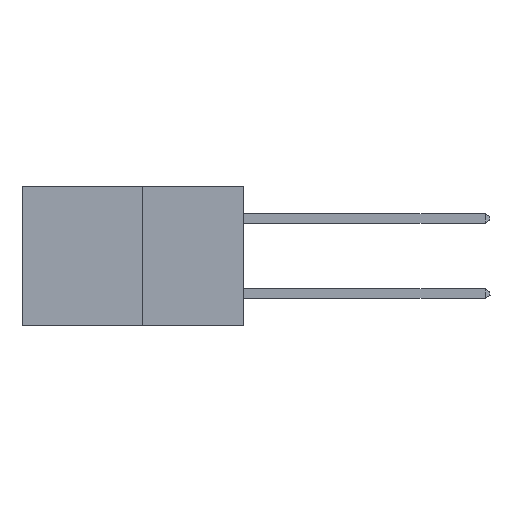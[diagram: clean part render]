
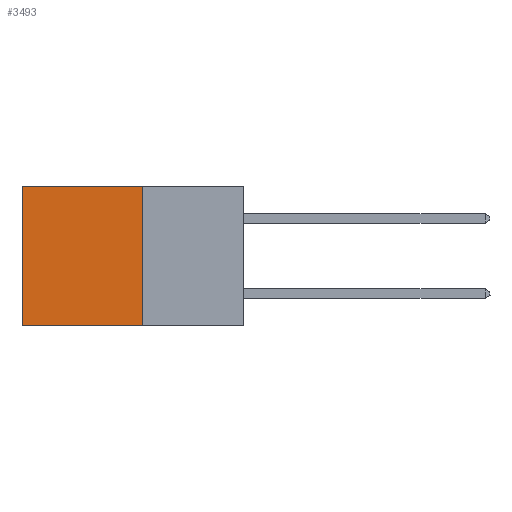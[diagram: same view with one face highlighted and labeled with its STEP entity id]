
A CAD part, left-side view. The second image highlights one B-rep face of the part: STEP entity #3493.
In plain terms, the highlighted planar face has unit normal (-1, 0, 0).
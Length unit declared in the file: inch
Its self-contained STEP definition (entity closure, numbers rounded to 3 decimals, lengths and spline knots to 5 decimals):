
#162 = EDGE_LOOP ( 'NONE', ( #3804, #6174, #7040, #8184 ) ) ;
#469 = CARTESIAN_POINT ( 'NONE',  ( 0.277, 0.27, 0. ) ) ;
#865 = EDGE_CURVE ( 'NONE', #2315, #2094, #4420, .T. ) ;
#960 = CARTESIAN_POINT ( 'NONE',  ( 0.277, 0.27, -0.37 ) ) ;
#1378 = EDGE_CURVE ( 'NONE', #2315, #7028, #4768, .T. ) ;
#1620 = LINE ( 'NONE', #10731, #13475 ) ;
#1769 = AXIS2_PLACEMENT_3D ( 'NONE', #960, #10136, #9156 ) ;
#1857 = VECTOR ( 'NONE', #6506, 39.37008 ) ;
#2094 = VERTEX_POINT ( 'NONE', #13293 ) ;
#2315 = VERTEX_POINT ( 'NONE', #469 ) ;
#2452 = EDGE_CURVE ( 'NONE', #7028, #11195, #1620, .T. ) ;
#2861 = PLANE ( 'NONE',  #1769 ) ;
#3493 = ADVANCED_FACE ( 'NONE', ( #5877 ), #2861, .F. ) ;
#3804 = ORIENTED_EDGE ( 'NONE', *, *, #2452, .T. ) ;
#4420 = LINE ( 'NONE', #10392, #9798 ) ;
#4768 = LINE ( 'NONE', #13107, #13834 ) ;
#5467 = CARTESIAN_POINT ( 'NONE',  ( 0.277, 0.27, -0.37 ) ) ;
#5877 = FACE_OUTER_BOUND ( 'NONE', #162, .T. ) ;
#6174 = ORIENTED_EDGE ( 'NONE', *, *, #13505, .F. ) ;
#6358 = DIRECTION ( 'NONE',  ( 0., 1., 0. ) ) ;
#6506 = DIRECTION ( 'NONE',  ( 0., 1., 0. ) ) ;
#7028 = VERTEX_POINT ( 'NONE', #10243 ) ;
#7040 = ORIENTED_EDGE ( 'NONE', *, *, #865, .F. ) ;
#7459 = LINE ( 'NONE', #5467, #1857 ) ;
#8127 = DIRECTION ( 'NONE',  ( 0., 0., -1. ) ) ;
#8184 = ORIENTED_EDGE ( 'NONE', *, *, #1378, .T. ) ;
#8373 = CARTESIAN_POINT ( 'NONE',  ( 0.277, 0.59, -0.37 ) ) ;
#9156 = DIRECTION ( 'NONE',  ( 0., 0., -1. ) ) ;
#9798 = VECTOR ( 'NONE', #11329, 39.37008 ) ;
#10136 = DIRECTION ( 'NONE',  ( 1., 0., 0. ) ) ;
#10243 = CARTESIAN_POINT ( 'NONE',  ( 0.277, 0.59, 0. ) ) ;
#10392 = CARTESIAN_POINT ( 'NONE',  ( 0.277, 0.27, -0.37 ) ) ;
#10731 = CARTESIAN_POINT ( 'NONE',  ( 0.277, 0.59, -0.37 ) ) ;
#11195 = VERTEX_POINT ( 'NONE', #8373 ) ;
#11329 = DIRECTION ( 'NONE',  ( 0., 0., -1. ) ) ;
#13107 = CARTESIAN_POINT ( 'NONE',  ( 0.277, 0.27, 0. ) ) ;
#13293 = CARTESIAN_POINT ( 'NONE',  ( 0.277, 0.27, -0.37 ) ) ;
#13475 = VECTOR ( 'NONE', #8127, 39.37008 ) ;
#13505 = EDGE_CURVE ( 'NONE', #2094, #11195, #7459, .T. ) ;
#13834 = VECTOR ( 'NONE', #6358, 39.37008 ) ;
